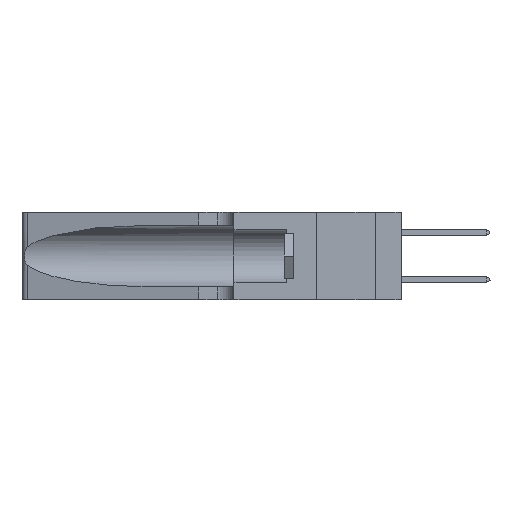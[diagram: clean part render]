
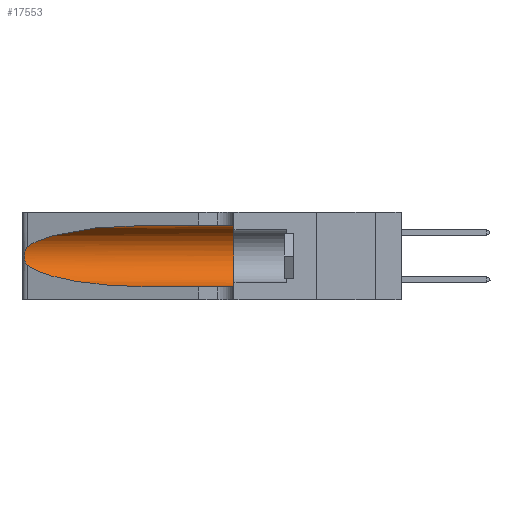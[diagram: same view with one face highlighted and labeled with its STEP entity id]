
A CAD part, left-side view. The second image highlights one B-rep face of the part: STEP entity #17553.
In plain terms, the highlighted cylindrical face has radius 3.308 mm (diameter 6.617 mm), a partial arc.
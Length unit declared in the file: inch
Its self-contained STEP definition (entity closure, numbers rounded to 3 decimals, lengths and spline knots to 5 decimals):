
#56 = AXIS2_PLACEMENT_3D ( 'NONE', #17118, #33000, #22345 ) ;
#266 = EDGE_CURVE ( 'NONE', #587, #15256, #18445, .T. ) ;
#320 = ORIENTED_EDGE ( 'NONE', *, *, #3576, .T. ) ;
#531 = ORIENTED_EDGE ( 'NONE', *, *, #23075, .T. ) ;
#587 = VERTEX_POINT ( 'NONE', #3359 ) ;
#1610 = CARTESIAN_POINT ( 'NONE',  ( 0.26075, 1.23896, 0.19203 ) ) ;
#2091 = CARTESIAN_POINT ( 'NONE',  ( 0.2373, 1.15595, 0.28018 ) ) ;
#2324 = EDGE_CURVE ( 'NONE', #27946, #4446, #20938, .T. ) ;
#2724 = CYLINDRICAL_SURFACE ( 'NONE', #56, 0.13025 ) ;
#3202 = CARTESIAN_POINT ( 'NONE',  ( 0.25487, 1.22718, 0.22369 ) ) ;
#3359 = CARTESIAN_POINT ( 'NONE',  ( 0.25487, 1.22718, 0.22369 ) ) ;
#3576 = EDGE_CURVE ( 'NONE', #34340, #587, #17392, .T. ) ;
#3807 = CARTESIAN_POINT ( 'NONE',  ( 0.1305, 0.72297, 0.31525 ) ) ;
#4237 = LINE ( 'NONE', #22126, #27178 ) ;
#4446 = VERTEX_POINT ( 'NONE', #9068 ) ;
#4556 = CARTESIAN_POINT ( 'NONE',  ( 0.26018, 1.23835, 0.19895 ) ) ;
#6374 = CARTESIAN_POINT ( 'NONE',  ( 0.25639, 1.23184, 0.21858 ) ) ;
#7253 = CARTESIAN_POINT ( 'NONE',  ( 0.18966, 0.96281, 0.05475 ) ) ;
#7730 = CARTESIAN_POINT ( 'NONE',  ( 0.1305, 0.72297, 0.05475 ) ) ;
#7929 = CARTESIAN_POINT ( 'NONE',  ( 0.25789, 1.23486, 0.15765 ) ) ;
#8033 = CARTESIAN_POINT ( 'NONE',  ( 0.25487, 1.22718, 0.14631 ) ) ;
#9068 = CARTESIAN_POINT ( 'NONE',  ( 0.1305, 0.35, 0.05475 ) ) ;
#11255 = LINE ( 'NONE', #32300, #22867 ) ;
#11458 = ORIENTED_EDGE ( 'NONE', *, *, #2324, .F. ) ;
#11548 = ORIENTED_EDGE ( 'NONE', *, *, #27617, .T. ) ;
#12817 = CARTESIAN_POINT ( 'NONE',  ( 0.1305, 0.35, 0.185 ) ) ;
#12985 = CARTESIAN_POINT ( 'NONE',  ( 0.25856, 1.23593, 0.16098 ) ) ;
#13018 = CARTESIAN_POINT ( 'NONE',  ( 0.25487, 1.22718, 0.14631 ) ) ;
#13039 = CARTESIAN_POINT ( 'NONE',  ( 0.1305, 0.72297, 0.31525 ) ) ;
#13158 = CARTESIAN_POINT ( 'NONE',  ( 0.25487, 1.22718, 0.22369 ) ) ;
#13732 = EDGE_LOOP ( 'NONE', ( #320, #29051, #531, #11548, #11458, #20340 ) ) ;
#14432 = CARTESIAN_POINT ( 'NONE',  ( 0.25854, 1.2359, 0.20912 ) ) ;
#15256 = VERTEX_POINT ( 'NONE', #8033 ) ;
#17118 = CARTESIAN_POINT ( 'NONE',  ( 0.1305, 1.61858, 0.185 ) ) ;
#17392 =( BOUNDED_CURVE ( )  B_SPLINE_CURVE ( 3, ( #13039, #18380, #2091, #13158 ),
 .UNSPECIFIED., .F., .F. ) 
 B_SPLINE_CURVE_WITH_KNOTS ( ( 4, 4 ),
 ( 1.5708, 2.84003 ),
 .UNSPECIFIED. ) 
 CURVE ( )  GEOMETRIC_REPRESENTATION_ITEM ( )  RATIONAL_B_SPLINE_CURVE ( ( 1., 0.87, 0.87, 1. ) ) 
 REPRESENTATION_ITEM ( '' )  );
#17553 = ADVANCED_FACE ( 'NONE', ( #31134 ), #2724, .F. ) ;
#18312 = VERTEX_POINT ( 'NONE', #25552 ) ;
#18380 = CARTESIAN_POINT ( 'NONE',  ( 0.18966, 0.96281, 0.31525 ) ) ;
#18445 = B_SPLINE_CURVE_WITH_KNOTS ( 'NONE', 3,
 ( #3202, #22364, #6374, #31329, #14432, #4556, #1610, #31279, #28641, #12985, #7929, #21344, #24016, #29125 ),
 .UNSPECIFIED., .F., .F.,
 ( 4, 2, 2, 2, 2, 2, 4 ),
 ( 0., 0.00027, 0.00053, 0.00107, 0.0016, 0.00187, 0.00214 ),
 .UNSPECIFIED. ) ;
#20340 = ORIENTED_EDGE ( 'NONE', *, *, #28865, .F. ) ;
#20938 = CIRCLE ( 'NONE', #31995, 0.13025 ) ;
#21344 = CARTESIAN_POINT ( 'NONE',  ( 0.25639, 1.23186, 0.15144 ) ) ;
#22126 = CARTESIAN_POINT ( 'NONE',  ( 0.1305, 1.61858, 0.31525 ) ) ;
#22345 = DIRECTION ( 'NONE',  ( 0., 0., -1. ) ) ;
#22364 = CARTESIAN_POINT ( 'NONE',  ( 0.25555, 1.22994, 0.2215 ) ) ;
#22867 = VECTOR ( 'NONE', #30025, 39.37008 ) ;
#23075 = EDGE_CURVE ( 'NONE', #15256, #18312, #25693, .T. ) ;
#24016 = CARTESIAN_POINT ( 'NONE',  ( 0.25555, 1.22993, 0.14849 ) ) ;
#25552 = CARTESIAN_POINT ( 'NONE',  ( 0.1305, 0.72297, 0.05475 ) ) ;
#25693 =( BOUNDED_CURVE ( )  B_SPLINE_CURVE ( 3, ( #13018, #31646, #7253, #7730 ),
 .UNSPECIFIED., .F., .T. ) 
 B_SPLINE_CURVE_WITH_KNOTS ( ( 4, 4 ),
 ( 3.44316, 4.71239 ),
 .UNSPECIFIED. ) 
 CURVE ( )  GEOMETRIC_REPRESENTATION_ITEM ( )  RATIONAL_B_SPLINE_CURVE ( ( 1., 0.87, 0.87, 1. ) ) 
 REPRESENTATION_ITEM ( '' )  );
#27178 = VECTOR ( 'NONE', #32654, 39.37008 ) ;
#27617 = EDGE_CURVE ( 'NONE', #18312, #4446, #11255, .T. ) ;
#27946 = VERTEX_POINT ( 'NONE', #30839 ) ;
#28503 = DIRECTION ( 'NONE',  ( 0., 1., 0. ) ) ;
#28641 = CARTESIAN_POINT ( 'NONE',  ( 0.26017, 1.23833, 0.17102 ) ) ;
#28845 = DIRECTION ( 'NONE',  ( 0., 0., 1. ) ) ;
#28865 = EDGE_CURVE ( 'NONE', #34340, #27946, #4237, .T. ) ;
#29051 = ORIENTED_EDGE ( 'NONE', *, *, #266, .T. ) ;
#29125 = CARTESIAN_POINT ( 'NONE',  ( 0.25487, 1.22718, 0.14631 ) ) ;
#30025 = DIRECTION ( 'NONE',  ( 0., -1., 0. ) ) ;
#30839 = CARTESIAN_POINT ( 'NONE',  ( 0.1305, 0.35, 0.31525 ) ) ;
#31134 = FACE_OUTER_BOUND ( 'NONE', #13732, .T. ) ;
#31279 = CARTESIAN_POINT ( 'NONE',  ( 0.26075, 1.23896, 0.178 ) ) ;
#31329 = CARTESIAN_POINT ( 'NONE',  ( 0.25787, 1.23484, 0.2124 ) ) ;
#31646 = CARTESIAN_POINT ( 'NONE',  ( 0.2373, 1.15595, 0.08982 ) ) ;
#31995 = AXIS2_PLACEMENT_3D ( 'NONE', #12817, #28503, #28845 ) ;
#32300 = CARTESIAN_POINT ( 'NONE',  ( 0.1305, 1.61858, 0.05475 ) ) ;
#32654 = DIRECTION ( 'NONE',  ( 0., -1., 0. ) ) ;
#33000 = DIRECTION ( 'NONE',  ( 0., -1., 0. ) ) ;
#34340 = VERTEX_POINT ( 'NONE', #3807 ) ;
